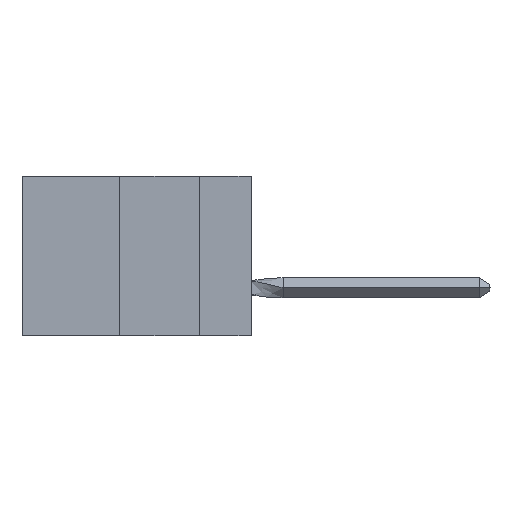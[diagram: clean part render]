
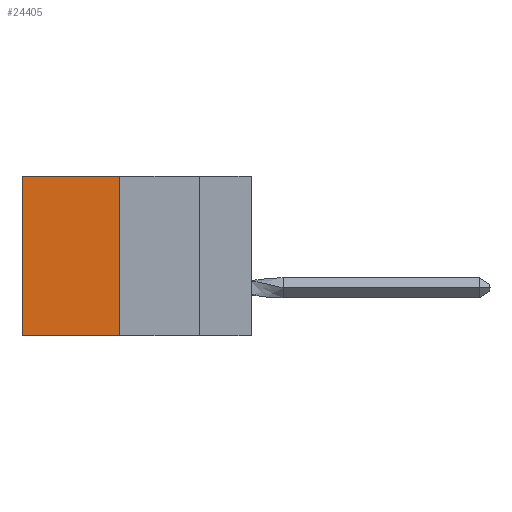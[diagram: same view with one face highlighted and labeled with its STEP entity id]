
A CAD part, left-side view. The second image highlights one B-rep face of the part: STEP entity #24405.
In plain terms, the highlighted planar face has unit normal (-1, 0, 0).
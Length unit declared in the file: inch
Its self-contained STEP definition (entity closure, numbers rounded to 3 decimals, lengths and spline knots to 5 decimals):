
#492 = CARTESIAN_POINT ( 'NONE',  ( 0.305, 0.413, -0.5 ) ) ;
#1380 = FACE_OUTER_BOUND ( 'NONE', #12179, .T. ) ;
#1500 = CARTESIAN_POINT ( 'NONE',  ( 0.305, 0.72, -0.5 ) ) ;
#2824 = DIRECTION ( 'NONE',  ( 0., 0., -1. ) ) ;
#3452 = LINE ( 'NONE', #18785, #13882 ) ;
#4063 = CARTESIAN_POINT ( 'NONE',  ( 0.305, 0.413, -0.5 ) ) ;
#4776 = AXIS2_PLACEMENT_3D ( 'NONE', #16631, #25489, #16552 ) ;
#4899 = DIRECTION ( 'NONE',  ( 0., 1., 0. ) ) ;
#5864 = DIRECTION ( 'NONE',  ( 0., 0., -1. ) ) ;
#7393 = ORIENTED_EDGE ( 'NONE', *, *, #21018, .T. ) ;
#8573 = VECTOR ( 'NONE', #4899, 39.37008 ) ;
#11309 = CARTESIAN_POINT ( 'NONE',  ( 0.305, 0.413, 0. ) ) ;
#11512 = CARTESIAN_POINT ( 'NONE',  ( 0.305, 0.413, -0.5 ) ) ;
#11679 = EDGE_CURVE ( 'NONE', #12807, #18246, #15792, .T. ) ;
#12179 = EDGE_LOOP ( 'NONE', ( #7393, #19934, #20085, #16632 ) ) ;
#12807 = VERTEX_POINT ( 'NONE', #12814 ) ;
#12814 = CARTESIAN_POINT ( 'NONE',  ( 0.305, 0.413, 0. ) ) ;
#13536 = DIRECTION ( 'NONE',  ( 0., 1., 0. ) ) ;
#13882 = VECTOR ( 'NONE', #5864, 39.37008 ) ;
#15684 = VERTEX_POINT ( 'NONE', #23192 ) ;
#15792 = LINE ( 'NONE', #492, #26561 ) ;
#16552 = DIRECTION ( 'NONE',  ( 0., 0., -1. ) ) ;
#16631 = CARTESIAN_POINT ( 'NONE',  ( 0.305, 0.413, -0.5 ) ) ;
#16632 = ORIENTED_EDGE ( 'NONE', *, *, #22317, .T. ) ;
#17771 = EDGE_CURVE ( 'NONE', #18246, #20238, #22987, .T. ) ;
#18246 = VERTEX_POINT ( 'NONE', #4063 ) ;
#18785 = CARTESIAN_POINT ( 'NONE',  ( 0.305, 0.72, -0.5 ) ) ;
#19010 = PLANE ( 'NONE',  #4776 ) ;
#19179 = VECTOR ( 'NONE', #13536, 39.37008 ) ;
#19934 = ORIENTED_EDGE ( 'NONE', *, *, #17771, .F. ) ;
#20085 = ORIENTED_EDGE ( 'NONE', *, *, #11679, .F. ) ;
#20238 = VERTEX_POINT ( 'NONE', #1500 ) ;
#21018 = EDGE_CURVE ( 'NONE', #15684, #20238, #3452, .T. ) ;
#22317 = EDGE_CURVE ( 'NONE', #12807, #15684, #22532, .T. ) ;
#22532 = LINE ( 'NONE', #11309, #19179 ) ;
#22987 = LINE ( 'NONE', #11512, #8573 ) ;
#23192 = CARTESIAN_POINT ( 'NONE',  ( 0.305, 0.72, 0. ) ) ;
#24405 = ADVANCED_FACE ( 'NONE', ( #1380 ), #19010, .F. ) ;
#25489 = DIRECTION ( 'NONE',  ( 1., 0., 0. ) ) ;
#26561 = VECTOR ( 'NONE', #2824, 39.37008 ) ;
